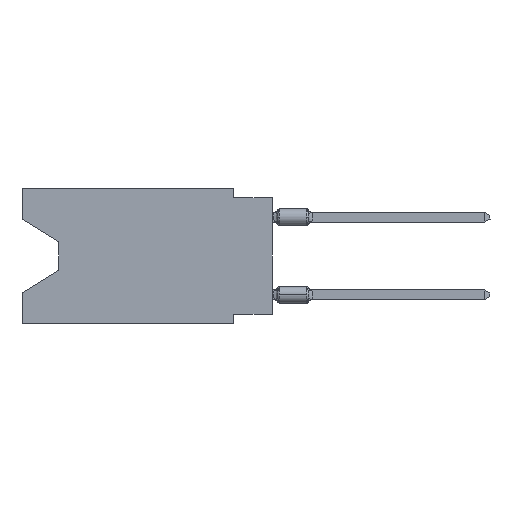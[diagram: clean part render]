
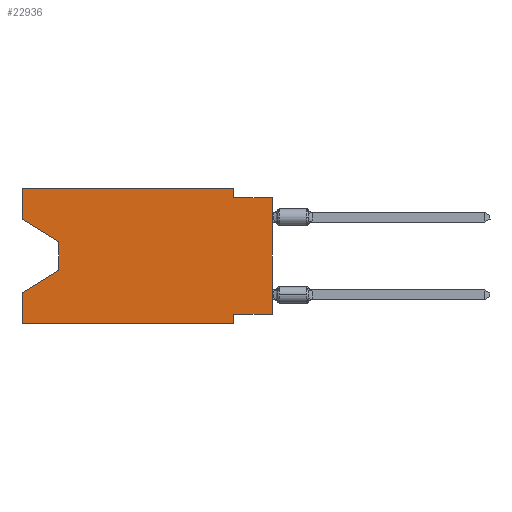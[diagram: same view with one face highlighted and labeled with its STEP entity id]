
A CAD part, left-side view. The second image highlights one B-rep face of the part: STEP entity #22936.
In plain terms, the highlighted planar face has unit normal (-1, 0, 0).
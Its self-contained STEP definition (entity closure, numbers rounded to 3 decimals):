
#56 = CARTESIAN_POINT ( 'NONE',  ( 0., 13.97, -3.505 ) ) ;
#83 = ORIENTED_EDGE ( 'NONE', *, *, #24931, .T. ) ;
#131 = EDGE_CURVE ( 'NONE', #45202, #7754, #25963, .T. ) ;
#250 = VERTEX_POINT ( 'NONE', #41282 ) ;
#330 = DIRECTION ( 'NONE',  ( 0., 0., 1. ) ) ;
#578 = LINE ( 'NONE', #14775, #44751 ) ;
#665 = ORIENTED_EDGE ( 'NONE', *, *, #26848, .T. ) ;
#1287 = DIRECTION ( 'NONE',  ( 0., 0., -1. ) ) ;
#1548 = CARTESIAN_POINT ( 'NONE',  ( 0., 2.54, -8.89 ) ) ;
#2630 = CARTESIAN_POINT ( 'NONE',  ( 0., 2.54, 0. ) ) ;
#4675 = VECTOR ( 'NONE', #24420, 1000. ) ;
#5929 = EDGE_CURVE ( 'NONE', #250, #13892, #26267, .T. ) ;
#6301 = DIRECTION ( 'NONE',  ( 0., 0., -1. ) ) ;
#6365 = CARTESIAN_POINT ( 'NONE',  ( 0., 16.383, 0. ) ) ;
#6625 = CARTESIAN_POINT ( 'NONE',  ( 0., 0., -8.255 ) ) ;
#7673 = CARTESIAN_POINT ( 'NONE',  ( 0., 0., -0.635 ) ) ;
#7707 = EDGE_CURVE ( 'NONE', #20986, #9868, #10792, .T. ) ;
#7754 = VERTEX_POINT ( 'NONE', #14745 ) ;
#8947 = DIRECTION ( 'NONE',  ( 1., 0., 0. ) ) ;
#9178 = EDGE_CURVE ( 'NONE', #44832, #13892, #38322, .T. ) ;
#9868 = VERTEX_POINT ( 'NONE', #37255 ) ;
#10792 = LINE ( 'NONE', #21046, #40273 ) ;
#11266 = EDGE_CURVE ( 'NONE', #44832, #26250, #14019, .T. ) ;
#11356 = DIRECTION ( 'NONE',  ( 0., 0., -1. ) ) ;
#11402 = CARTESIAN_POINT ( 'NONE',  ( 0., 16.383, -2.038 ) ) ;
#12720 = LINE ( 'NONE', #26908, #33460 ) ;
#13027 = CARTESIAN_POINT ( 'NONE',  ( 0., 13.97, -5.385 ) ) ;
#13053 = ORIENTED_EDGE ( 'NONE', *, *, #35145, .T. ) ;
#13892 = VERTEX_POINT ( 'NONE', #20003 ) ;
#14019 = LINE ( 'NONE', #30789, #22905 ) ;
#14745 = CARTESIAN_POINT ( 'NONE',  ( 0., 13.97, -5.385 ) ) ;
#14775 = CARTESIAN_POINT ( 'NONE',  ( 0., 16.383, 0. ) ) ;
#15135 = LINE ( 'NONE', #11402, #41519 ) ;
#16945 = ORIENTED_EDGE ( 'NONE', *, *, #9178, .T. ) ;
#18098 = CARTESIAN_POINT ( 'NONE',  ( 0., 16.383, -8.89 ) ) ;
#18113 = CARTESIAN_POINT ( 'NONE',  ( 0., 2.54, 0. ) ) ;
#20003 = CARTESIAN_POINT ( 'NONE',  ( 0., 0., -0.635 ) ) ;
#20027 = VECTOR ( 'NONE', #1287, 1000. ) ;
#20637 = LINE ( 'NONE', #45073, #23041 ) ;
#20641 = CARTESIAN_POINT ( 'NONE',  ( 0., 0., 0. ) ) ;
#20986 = VERTEX_POINT ( 'NONE', #18098 ) ;
#21046 = CARTESIAN_POINT ( 'NONE',  ( 0., 16.383, 0. ) ) ;
#21119 = ORIENTED_EDGE ( 'NONE', *, *, #5929, .F. ) ;
#21306 = DIRECTION ( 'NONE',  ( 0., -1., 0. ) ) ;
#21677 = EDGE_LOOP ( 'NONE', ( #83, #23374, #13053, #27942, #665, #25506, #34627, #16945, #21119, #39180, #30436, #39721 ) ) ;
#22350 = DIRECTION ( 'NONE',  ( 0., -0.855, -0.519 ) ) ;
#22905 = VECTOR ( 'NONE', #27765, 1000. ) ;
#22936 = ADVANCED_FACE ( 'NONE', ( #23592 ), #40813, .F. ) ;
#23041 = VECTOR ( 'NONE', #27384, 1000. ) ;
#23374 = ORIENTED_EDGE ( 'NONE', *, *, #131, .T. ) ;
#23566 = AXIS2_PLACEMENT_3D ( 'NONE', #6365, #8947, #30576 ) ;
#23592 = FACE_OUTER_BOUND ( 'NONE', #21677, .T. ) ;
#24143 = DIRECTION ( 'NONE',  ( 0., 0., 1. ) ) ;
#24420 = DIRECTION ( 'NONE',  ( 0., 0.855, -0.519 ) ) ;
#24931 = EDGE_CURVE ( 'NONE', #40683, #45202, #15135, .T. ) ;
#25206 = CARTESIAN_POINT ( 'NONE',  ( 0., 2.54, -8.255 ) ) ;
#25506 = ORIENTED_EDGE ( 'NONE', *, *, #33975, .F. ) ;
#25963 = LINE ( 'NONE', #29235, #20027 ) ;
#26250 = VERTEX_POINT ( 'NONE', #25206 ) ;
#26267 = LINE ( 'NONE', #7673, #40107 ) ;
#26848 = EDGE_CURVE ( 'NONE', #20986, #33034, #12720, .T. ) ;
#26908 = CARTESIAN_POINT ( 'NONE',  ( 0., 16.383, -8.89 ) ) ;
#27017 = CARTESIAN_POINT ( 'NONE',  ( 0., 2.54, -8.89 ) ) ;
#27384 = DIRECTION ( 'NONE',  ( 0., -1., 0. ) ) ;
#27765 = DIRECTION ( 'NONE',  ( 0., 1., 0. ) ) ;
#27942 = ORIENTED_EDGE ( 'NONE', *, *, #7707, .F. ) ;
#29235 = CARTESIAN_POINT ( 'NONE',  ( 0., 13.97, -3.505 ) ) ;
#30064 = VERTEX_POINT ( 'NONE', #2630 ) ;
#30436 = ORIENTED_EDGE ( 'NONE', *, *, #31600, .F. ) ;
#30576 = DIRECTION ( 'NONE',  ( 0., 0., -1. ) ) ;
#30789 = CARTESIAN_POINT ( 'NONE',  ( 0., 0., -8.255 ) ) ;
#31600 = EDGE_CURVE ( 'NONE', #45377, #30064, #20637, .T. ) ;
#31627 = LINE ( 'NONE', #13027, #4675 ) ;
#33034 = VERTEX_POINT ( 'NONE', #1548 ) ;
#33460 = VECTOR ( 'NONE', #21306, 1000. ) ;
#33975 = EDGE_CURVE ( 'NONE', #26250, #33034, #33980, .T. ) ;
#33980 = LINE ( 'NONE', #27017, #42500 ) ;
#34627 = ORIENTED_EDGE ( 'NONE', *, *, #11266, .F. ) ;
#34629 = EDGE_CURVE ( 'NONE', #40683, #45377, #578, .T. ) ;
#35145 = EDGE_CURVE ( 'NONE', #7754, #9868, #31627, .T. ) ;
#36791 = CARTESIAN_POINT ( 'NONE',  ( 0., 16.383, 0. ) ) ;
#37018 = VECTOR ( 'NONE', #11356, 1000. ) ;
#37255 = CARTESIAN_POINT ( 'NONE',  ( 0., 16.383, -6.852 ) ) ;
#38322 = LINE ( 'NONE', #20641, #43630 ) ;
#39180 = ORIENTED_EDGE ( 'NONE', *, *, #41901, .F. ) ;
#39721 = ORIENTED_EDGE ( 'NONE', *, *, #34629, .F. ) ;
#40107 = VECTOR ( 'NONE', #40456, 1000. ) ;
#40144 = CARTESIAN_POINT ( 'NONE',  ( 0., 16.383, -2.038 ) ) ;
#40273 = VECTOR ( 'NONE', #330, 1000. ) ;
#40456 = DIRECTION ( 'NONE',  ( 0., -1., 0. ) ) ;
#40683 = VERTEX_POINT ( 'NONE', #40144 ) ;
#40813 = PLANE ( 'NONE',  #23566 ) ;
#41282 = CARTESIAN_POINT ( 'NONE',  ( 0., 2.54, -0.635 ) ) ;
#41519 = VECTOR ( 'NONE', #22350, 1000. ) ;
#41901 = EDGE_CURVE ( 'NONE', #30064, #250, #43235, .T. ) ;
#42500 = VECTOR ( 'NONE', #6301, 1000. ) ;
#43165 = DIRECTION ( 'NONE',  ( 0., 0., 1. ) ) ;
#43235 = LINE ( 'NONE', #18113, #37018 ) ;
#43630 = VECTOR ( 'NONE', #24143, 1000. ) ;
#44751 = VECTOR ( 'NONE', #43165, 1000. ) ;
#44832 = VERTEX_POINT ( 'NONE', #6625 ) ;
#45073 = CARTESIAN_POINT ( 'NONE',  ( 0., 16.383, 0. ) ) ;
#45202 = VERTEX_POINT ( 'NONE', #56 ) ;
#45377 = VERTEX_POINT ( 'NONE', #36791 ) ;
